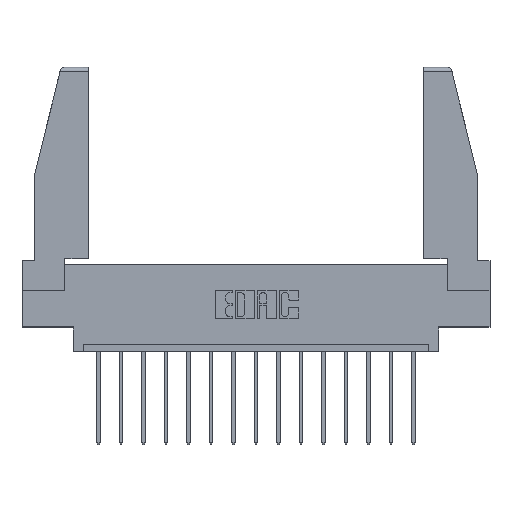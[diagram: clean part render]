
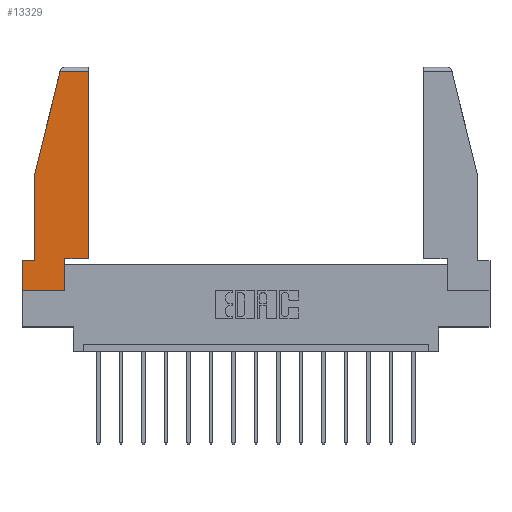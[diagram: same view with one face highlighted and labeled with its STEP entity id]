
A CAD part, top view. The second image highlights one B-rep face of the part: STEP entity #13329.
In plain terms, the highlighted planar face has unit normal (0, 0, 1).
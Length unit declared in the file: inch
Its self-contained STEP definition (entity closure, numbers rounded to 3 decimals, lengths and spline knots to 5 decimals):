
#70 = FACE_OUTER_BOUND ( 'NONE', #15380, .T. ) ;
#128 = VECTOR ( 'NONE', #13319, 39.37008 ) ;
#314 = CARTESIAN_POINT ( 'NONE',  ( 0., 0.21, 0. ) ) ;
#407 = EDGE_CURVE ( 'NONE', #16197, #7049, #10424, .T. ) ;
#475 = LINE ( 'NONE', #1978, #900 ) ;
#502 = DIRECTION ( 'NONE',  ( 0., -1., 0. ) ) ;
#807 = CARTESIAN_POINT ( 'NONE',  ( 0.271, 1.55, 0. ) ) ;
#900 = VECTOR ( 'NONE', #7237, 39.37008 ) ;
#902 = EDGE_CURVE ( 'NONE', #10904, #9317, #12265, .T. ) ;
#1210 = VERTEX_POINT ( 'NONE', #6231 ) ;
#1440 = ORIENTED_EDGE ( 'NONE', *, *, #3363, .T. ) ;
#1978 = CARTESIAN_POINT ( 'NONE',  ( 0., 0., 0. ) ) ;
#2102 = VERTEX_POINT ( 'NONE', #6926 ) ;
#2582 = VECTOR ( 'NONE', #6206, 39.37008 ) ;
#3218 = EDGE_CURVE ( 'NONE', #7049, #6084, #15891, .T. ) ;
#3363 = EDGE_CURVE ( 'NONE', #6084, #1210, #4869, .T. ) ;
#3424 = EDGE_CURVE ( 'NONE', #1210, #2102, #475, .T. ) ;
#3482 = AXIS2_PLACEMENT_3D ( 'NONE', #10348, #7585, #5020 ) ;
#3541 = LINE ( 'NONE', #10913, #10032 ) ;
#3562 = ORIENTED_EDGE ( 'NONE', *, *, #3424, .T. ) ;
#4239 = CARTESIAN_POINT ( 'NONE',  ( 0.461, 0.223, 0. ) ) ;
#4286 = ORIENTED_EDGE ( 'NONE', *, *, #902, .T. ) ;
#4470 = CARTESIAN_POINT ( 'NONE',  ( 0.086, 0.8, 0. ) ) ;
#4724 = DIRECTION ( 'NONE',  ( -0.239, -0.971, 0. ) ) ;
#4815 = EDGE_CURVE ( 'NONE', #2102, #5404, #3541, .T. ) ;
#4869 = LINE ( 'NONE', #314, #11715 ) ;
#4966 = ORIENTED_EDGE ( 'NONE', *, *, #7853, .T. ) ;
#5020 = DIRECTION ( 'NONE',  ( 1., 0., 0. ) ) ;
#5404 = VERTEX_POINT ( 'NONE', #12892 ) ;
#5868 = CARTESIAN_POINT ( 'NONE',  ( 0.086, 0.8, 0. ) ) ;
#6084 = VERTEX_POINT ( 'NONE', #6184 ) ;
#6184 = CARTESIAN_POINT ( 'NONE',  ( 0., 0.21, 0. ) ) ;
#6206 = DIRECTION ( 'NONE',  ( -1., 0., 0. ) ) ;
#6231 = CARTESIAN_POINT ( 'NONE',  ( 0., 0., 0. ) ) ;
#6455 = VECTOR ( 'NONE', #502, 39.37008 ) ;
#6853 = DIRECTION ( 'NONE',  ( 0., 1., 0. ) ) ;
#6879 = VECTOR ( 'NONE', #8256, 39.37008 ) ;
#6904 = CARTESIAN_POINT ( 'NONE',  ( 0.297, 0.223, 0. ) ) ;
#6926 = CARTESIAN_POINT ( 'NONE',  ( 0.297, 0., 0. ) ) ;
#7049 = VERTEX_POINT ( 'NONE', #12231 ) ;
#7068 = EDGE_CURVE ( 'NONE', #5404, #10904, #8913, .T. ) ;
#7237 = DIRECTION ( 'NONE',  ( 1., 0., 0. ) ) ;
#7370 = DIRECTION ( 'NONE',  ( -1., 0., 0. ) ) ;
#7585 = DIRECTION ( 'NONE',  ( 0., 0., 1. ) ) ;
#7853 = EDGE_CURVE ( 'NONE', #11863, #16197, #9934, .T. ) ;
#8256 = DIRECTION ( 'NONE',  ( 0., 1., 0. ) ) ;
#8578 = CARTESIAN_POINT ( 'NONE',  ( 0.461, 1.52, 0. ) ) ;
#8913 = LINE ( 'NONE', #6904, #128 ) ;
#9317 = VERTEX_POINT ( 'NONE', #8578 ) ;
#9527 = ORIENTED_EDGE ( 'NONE', *, *, #407, .T. ) ;
#9710 = LINE ( 'NONE', #15615, #2582 ) ;
#9762 = CARTESIAN_POINT ( 'NONE',  ( 0.2636, 1.52, 0. ) ) ;
#9804 = ORIENTED_EDGE ( 'NONE', *, *, #4815, .T. ) ;
#9934 = LINE ( 'NONE', #807, #13451 ) ;
#10032 = VECTOR ( 'NONE', #6853, 39.37008 ) ;
#10082 = ORIENTED_EDGE ( 'NONE', *, *, #13280, .T. ) ;
#10348 = CARTESIAN_POINT ( 'NONE',  ( 0., 0., 0. ) ) ;
#10424 = LINE ( 'NONE', #4470, #6455 ) ;
#10904 = VERTEX_POINT ( 'NONE', #14444 ) ;
#10913 = CARTESIAN_POINT ( 'NONE',  ( 0.297, 0., 0. ) ) ;
#10920 = ORIENTED_EDGE ( 'NONE', *, *, #3218, .T. ) ;
#11715 = VECTOR ( 'NONE', #12141, 39.37008 ) ;
#11863 = VERTEX_POINT ( 'NONE', #9762 ) ;
#12141 = DIRECTION ( 'NONE',  ( 0., -1., 0. ) ) ;
#12231 = CARTESIAN_POINT ( 'NONE',  ( 0.086, 0.21, 0. ) ) ;
#12265 = LINE ( 'NONE', #4239, #6879 ) ;
#12678 = CARTESIAN_POINT ( 'NONE',  ( 0., 0.21, 0. ) ) ;
#12892 = CARTESIAN_POINT ( 'NONE',  ( 0.297, 0.223, 0. ) ) ;
#13280 = EDGE_CURVE ( 'NONE', #9317, #11863, #9710, .T. ) ;
#13319 = DIRECTION ( 'NONE',  ( 1., 0., 0. ) ) ;
#13329 = ADVANCED_FACE ( 'NONE', ( #70 ), #15497, .T. ) ;
#13451 = VECTOR ( 'NONE', #4724, 39.37008 ) ;
#14444 = CARTESIAN_POINT ( 'NONE',  ( 0.461, 0.223, 0. ) ) ;
#15064 = VECTOR ( 'NONE', #7370, 39.37008 ) ;
#15380 = EDGE_LOOP ( 'NONE', ( #4286, #10082, #4966, #9527, #10920, #1440, #3562, #9804, #15698 ) ) ;
#15497 = PLANE ( 'NONE',  #3482 ) ;
#15615 = CARTESIAN_POINT ( 'NONE',  ( 0., 1.52, 0. ) ) ;
#15698 = ORIENTED_EDGE ( 'NONE', *, *, #7068, .T. ) ;
#15891 = LINE ( 'NONE', #12678, #15064 ) ;
#16197 = VERTEX_POINT ( 'NONE', #5868 ) ;
